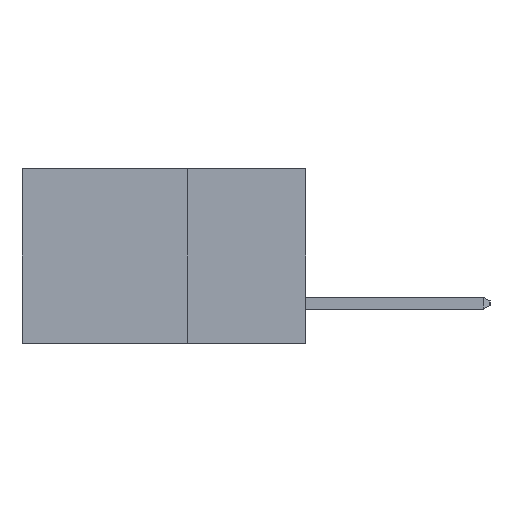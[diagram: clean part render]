
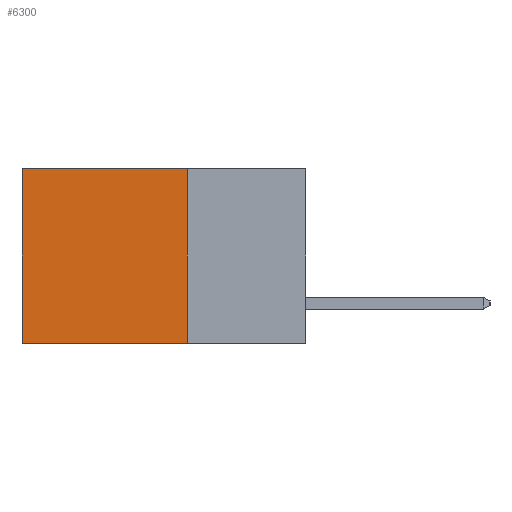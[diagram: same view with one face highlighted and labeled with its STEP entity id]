
A CAD part, left-side view. The second image highlights one B-rep face of the part: STEP entity #6300.
In plain terms, the highlighted planar face has unit normal (-1, 0, 0).
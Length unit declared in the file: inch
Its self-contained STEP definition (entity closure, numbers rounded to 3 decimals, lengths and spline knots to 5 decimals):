
#50 = CARTESIAN_POINT ( 'NONE',  ( 0.298, 0.25, -0.37 ) ) ;
#268 = LINE ( 'NONE', #3098, #4410 ) ;
#351 = EDGE_LOOP ( 'NONE', ( #5581, #8356, #4288, #10055 ) ) ;
#396 = CARTESIAN_POINT ( 'NONE',  ( 0.298, 0.6, 0. ) ) ;
#468 = CARTESIAN_POINT ( 'NONE',  ( 0.298, 0.6, -0.37 ) ) ;
#714 = EDGE_CURVE ( 'NONE', #8532, #3460, #8120, .T. ) ;
#1453 = DIRECTION ( 'NONE',  ( 0., 1., 0. ) ) ;
#1506 = CARTESIAN_POINT ( 'NONE',  ( 0.298, 0.6, 0. ) ) ;
#1585 = VECTOR ( 'NONE', #4987, 39.37008 ) ;
#2700 = DIRECTION ( 'NONE',  ( 0., 1., 0. ) ) ;
#3098 = CARTESIAN_POINT ( 'NONE',  ( 0.298, 0.25, -0.37 ) ) ;
#3155 = VERTEX_POINT ( 'NONE', #468 ) ;
#3460 = VERTEX_POINT ( 'NONE', #50 ) ;
#3810 = CARTESIAN_POINT ( 'NONE',  ( 0.298, 0.25, 0. ) ) ;
#4288 = ORIENTED_EDGE ( 'NONE', *, *, #714, .F. ) ;
#4410 = VECTOR ( 'NONE', #1453, 39.37008 ) ;
#4630 = PLANE ( 'NONE',  #7697 ) ;
#4877 = VECTOR ( 'NONE', #2700, 39.37008 ) ;
#4987 = DIRECTION ( 'NONE',  ( 0., 0., -1. ) ) ;
#5390 = VECTOR ( 'NONE', #8980, 39.37008 ) ;
#5476 = DIRECTION ( 'NONE',  ( 0., 0., -1. ) ) ;
#5581 = ORIENTED_EDGE ( 'NONE', *, *, #5943, .T. ) ;
#5943 = EDGE_CURVE ( 'NONE', #8845, #3155, #7786, .T. ) ;
#6300 = ADVANCED_FACE ( 'NONE', ( #10209 ), #4630, .F. ) ;
#7697 = AXIS2_PLACEMENT_3D ( 'NONE', #3810, #10097, #5476 ) ;
#7786 = LINE ( 'NONE', #1506, #5390 ) ;
#8120 = LINE ( 'NONE', #9957, #1585 ) ;
#8356 = ORIENTED_EDGE ( 'NONE', *, *, #9055, .F. ) ;
#8532 = VERTEX_POINT ( 'NONE', #9612 ) ;
#8845 = VERTEX_POINT ( 'NONE', #396 ) ;
#8980 = DIRECTION ( 'NONE',  ( 0., 0., -1. ) ) ;
#9055 = EDGE_CURVE ( 'NONE', #3460, #3155, #268, .T. ) ;
#9108 = LINE ( 'NONE', #9153, #4877 ) ;
#9153 = CARTESIAN_POINT ( 'NONE',  ( 0.298, 0.25, 0. ) ) ;
#9612 = CARTESIAN_POINT ( 'NONE',  ( 0.298, 0.25, 0. ) ) ;
#9957 = CARTESIAN_POINT ( 'NONE',  ( 0.298, 0.25, 0. ) ) ;
#10051 = EDGE_CURVE ( 'NONE', #8532, #8845, #9108, .T. ) ;
#10055 = ORIENTED_EDGE ( 'NONE', *, *, #10051, .T. ) ;
#10097 = DIRECTION ( 'NONE',  ( 1., 0., 0. ) ) ;
#10209 = FACE_OUTER_BOUND ( 'NONE', #351, .T. ) ;
